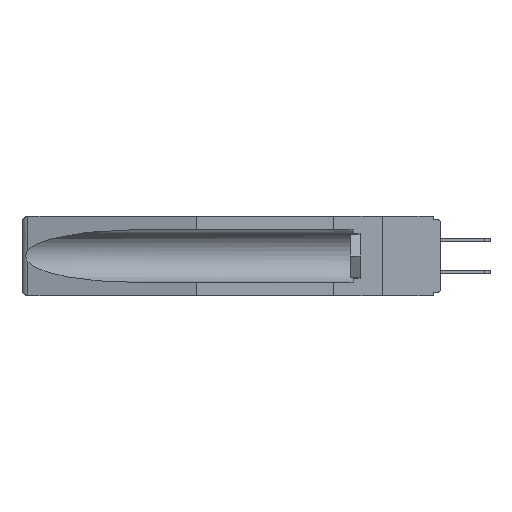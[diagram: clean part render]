
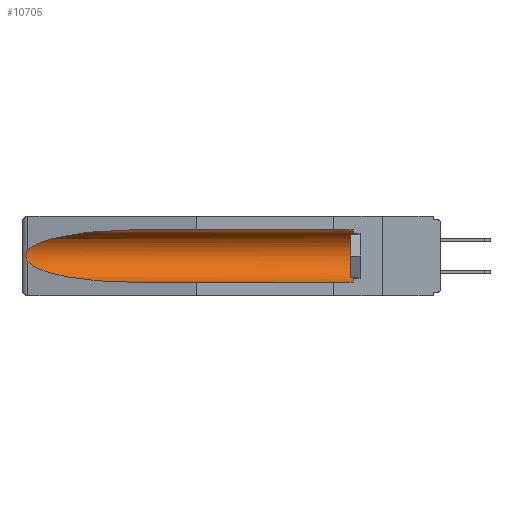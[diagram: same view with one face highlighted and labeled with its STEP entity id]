
A CAD part, left-side view. The second image highlights one B-rep face of the part: STEP entity #10705.
In plain terms, the highlighted cylindrical face has radius 2.857 mm (diameter 5.715 mm), a partial arc.
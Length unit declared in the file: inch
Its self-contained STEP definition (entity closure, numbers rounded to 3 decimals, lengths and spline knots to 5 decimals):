
#642 = CARTESIAN_POINT ( 'NONE',  ( 0.155, 1.07973, -0.284 ) ) ;
#707 = ORIENTED_EDGE ( 'NONE', *, *, #1596, .T. ) ;
#816 = EDGE_CURVE ( 'NONE', #7937, #15194, #13666, .T. ) ;
#1005 = EDGE_LOOP ( 'NONE', ( #707, #13522, #13266, #9577, #6481, #8752 ) ) ;
#1490 = CARTESIAN_POINT ( 'NONE',  ( 0.155, -0.30754, -0.284 ) ) ;
#1596 = EDGE_CURVE ( 'NONE', #4632, #17972, #4015, .T. ) ;
#1979 = CARTESIAN_POINT ( 'NONE',  ( 0.155, 1.07973, -0.059 ) ) ;
#3445 = DIRECTION ( 'NONE',  ( 0., -1., 0. ) ) ;
#3765 = CARTESIAN_POINT ( 'NONE',  ( 0.26537, 1.52718, -0.19328 ) ) ;
#3893 = CARTESIAN_POINT ( 'NONE',  ( 0.26655, 1.53094, -0.18657 ) ) ;
#4015 =( BOUNDED_CURVE ( )  B_SPLINE_CURVE ( 3, ( #6595, #19144, #12755, #15982 ),
 .UNSPECIFIED., .F., .F. ) 
 B_SPLINE_CURVE_WITH_KNOTS ( ( 4, 4 ),
 ( 4.71239, 6.08839 ),
 .UNSPECIFIED. ) 
 CURVE ( )  GEOMETRIC_REPRESENTATION_ITEM ( )  RATIONAL_B_SPLINE_CURVE ( ( 1., 0.848, 0.848, 1. ) ) 
 REPRESENTATION_ITEM ( '' )  );
#4632 = VERTEX_POINT ( 'NONE', #1979 ) ;
#4899 = B_SPLINE_CURVE_WITH_KNOTS ( 'NONE', 3,
 ( #15316, #5717, #13580, #5572, #8820, #10639, #20092, #3893, #20159, #18388 ),
 .UNSPECIFIED., .F., .F.,
 ( 4, 2, 2, 2, 4 ),
 ( 0., 0.00029, 0.00058, 0.00087, 0.00117 ),
 .UNSPECIFIED. ) ;
#4999 = AXIS2_PLACEMENT_3D ( 'NONE', #19520, #3445, #7375 ) ;
#5572 = CARTESIAN_POINT ( 'NONE',  ( 0.2673, 1.5327, -0.16383 ) ) ;
#5681 = CARTESIAN_POINT ( 'NONE',  ( 0.155, -0.30754, -0.059 ) ) ;
#5717 = CARTESIAN_POINT ( 'NONE',  ( 0.26597, 1.52961, -0.15275 ) ) ;
#5924 = CARTESIAN_POINT ( 'NONE',  ( 0.155, 0.126, -0.059 ) ) ;
#6446 = CARTESIAN_POINT ( 'NONE',  ( 0.26537, 1.52718, -0.19328 ) ) ;
#6481 = ORIENTED_EDGE ( 'NONE', *, *, #816, .T. ) ;
#6595 = CARTESIAN_POINT ( 'NONE',  ( 0.155, 1.07973, -0.059 ) ) ;
#6693 = CARTESIAN_POINT ( 'NONE',  ( 0.155, 0.126, -0.284 ) ) ;
#6992 = EDGE_CURVE ( 'NONE', #17482, #19255, #17058, .T. ) ;
#7375 = DIRECTION ( 'NONE',  ( 0., 0., 1. ) ) ;
#7937 = VERTEX_POINT ( 'NONE', #6693 ) ;
#8141 = EDGE_CURVE ( 'NONE', #17972, #17482, #4899, .T. ) ;
#8495 = CARTESIAN_POINT ( 'NONE',  ( 0.21114, 1.30732, -0.284 ) ) ;
#8706 = AXIS2_PLACEMENT_3D ( 'NONE', #19730, #16703, #15158 ) ;
#8752 = ORIENTED_EDGE ( 'NONE', *, *, #16669, .T. ) ;
#8820 = CARTESIAN_POINT ( 'NONE',  ( 0.2675, 1.53308, -0.16763 ) ) ;
#9373 = LINE ( 'NONE', #5681, #20236 ) ;
#9577 = ORIENTED_EDGE ( 'NONE', *, *, #19080, .F. ) ;
#10046 = VECTOR ( 'NONE', #17720, 39.37008 ) ;
#10639 = CARTESIAN_POINT ( 'NONE',  ( 0.2675, 1.53308, -0.17534 ) ) ;
#10705 = ADVANCED_FACE ( 'NONE', ( #18940 ), #11147, .F. ) ;
#11147 = CYLINDRICAL_SURFACE ( 'NONE', #8706, 0.1125 ) ;
#12755 = CARTESIAN_POINT ( 'NONE',  ( 0.25451, 1.48313, -0.09465 ) ) ;
#12842 = LINE ( 'NONE', #1490, #10046 ) ;
#13044 = CARTESIAN_POINT ( 'NONE',  ( 0.155, 1.07973, -0.284 ) ) ;
#13266 = ORIENTED_EDGE ( 'NONE', *, *, #6992, .T. ) ;
#13522 = ORIENTED_EDGE ( 'NONE', *, *, #8141, .T. ) ;
#13580 = CARTESIAN_POINT ( 'NONE',  ( 0.26654, 1.53092, -0.15636 ) ) ;
#13666 = CIRCLE ( 'NONE', #4999, 0.1125 ) ;
#15158 = DIRECTION ( 'NONE',  ( 0., 0., 1. ) ) ;
#15194 = VERTEX_POINT ( 'NONE', #5924 ) ;
#15316 = CARTESIAN_POINT ( 'NONE',  ( 0.26537, 1.52718, -0.14972 ) ) ;
#15349 = DIRECTION ( 'NONE',  ( 0., 1., 0. ) ) ;
#15982 = CARTESIAN_POINT ( 'NONE',  ( 0.26537, 1.52718, -0.14972 ) ) ;
#16669 = EDGE_CURVE ( 'NONE', #15194, #4632, #9373, .T. ) ;
#16703 = DIRECTION ( 'NONE',  ( 0., 1., 0. ) ) ;
#17058 =( BOUNDED_CURVE ( )  B_SPLINE_CURVE ( 3, ( #3765, #18130, #8495, #642 ),
 .UNSPECIFIED., .F., .F. ) 
 B_SPLINE_CURVE_WITH_KNOTS ( ( 4, 4 ),
 ( 0.1948, 1.5708 ),
 .UNSPECIFIED. ) 
 CURVE ( )  GEOMETRIC_REPRESENTATION_ITEM ( )  RATIONAL_B_SPLINE_CURVE ( ( 1., 0.848, 0.848, 1. ) ) 
 REPRESENTATION_ITEM ( '' )  );
#17482 = VERTEX_POINT ( 'NONE', #6446 ) ;
#17720 = DIRECTION ( 'NONE',  ( 0., 1., 0. ) ) ;
#17972 = VERTEX_POINT ( 'NONE', #17995 ) ;
#17995 = CARTESIAN_POINT ( 'NONE',  ( 0.26537, 1.52718, -0.14972 ) ) ;
#18130 = CARTESIAN_POINT ( 'NONE',  ( 0.25451, 1.48313, -0.24835 ) ) ;
#18388 = CARTESIAN_POINT ( 'NONE',  ( 0.26537, 1.52718, -0.19328 ) ) ;
#18940 = FACE_OUTER_BOUND ( 'NONE', #1005, .T. ) ;
#19080 = EDGE_CURVE ( 'NONE', #7937, #19255, #12842, .T. ) ;
#19144 = CARTESIAN_POINT ( 'NONE',  ( 0.21114, 1.30732, -0.059 ) ) ;
#19255 = VERTEX_POINT ( 'NONE', #13044 ) ;
#19520 = CARTESIAN_POINT ( 'NONE',  ( 0.155, 0.126, -0.1715 ) ) ;
#19730 = CARTESIAN_POINT ( 'NONE',  ( 0.155, -0.30754, -0.1715 ) ) ;
#20092 = CARTESIAN_POINT ( 'NONE',  ( 0.2673, 1.53269, -0.17917 ) ) ;
#20159 = CARTESIAN_POINT ( 'NONE',  ( 0.26597, 1.5296, -0.19026 ) ) ;
#20236 = VECTOR ( 'NONE', #15349, 39.37008 ) ;
